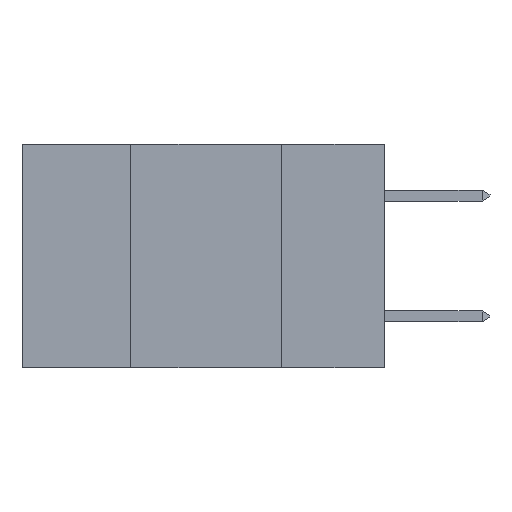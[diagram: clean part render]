
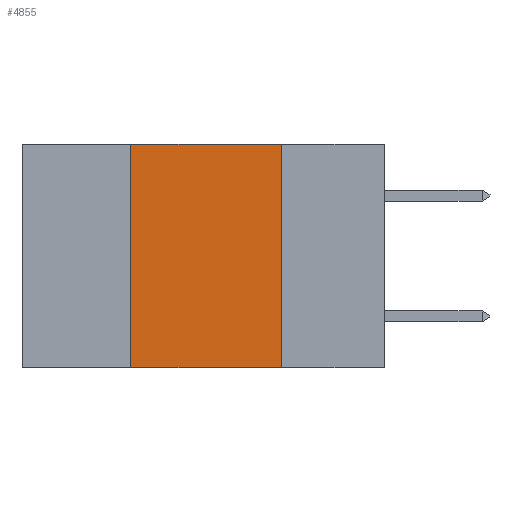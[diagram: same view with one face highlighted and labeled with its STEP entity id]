
A CAD part, left-side view. The second image highlights one B-rep face of the part: STEP entity #4855.
In plain terms, the highlighted planar face has unit normal (-1, 0, 0).
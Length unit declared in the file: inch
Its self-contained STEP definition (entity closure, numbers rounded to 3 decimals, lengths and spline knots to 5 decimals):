
#382 = CARTESIAN_POINT ( 'NONE',  ( 0., 0.42, -0.37 ) ) ;
#876 = VECTOR ( 'NONE', #8269, 39.37008 ) ;
#1705 = AXIS2_PLACEMENT_3D ( 'NONE', #3539, #5589, #12996 ) ;
#2665 = EDGE_CURVE ( 'NONE', #5939, #7210, #4431, .T. ) ;
#2969 = ORIENTED_EDGE ( 'NONE', *, *, #2665, .F. ) ;
#3015 = ORIENTED_EDGE ( 'NONE', *, *, #3837, .F. ) ;
#3060 = ORIENTED_EDGE ( 'NONE', *, *, #10704, .F. ) ;
#3158 = ORIENTED_EDGE ( 'NONE', *, *, #7846, .T. ) ;
#3539 = CARTESIAN_POINT ( 'NONE',  ( 0., 0.6, 0. ) ) ;
#3681 = LINE ( 'NONE', #5113, #876 ) ;
#3837 = EDGE_CURVE ( 'NONE', #6225, #5939, #9857, .T. ) ;
#4431 = LINE ( 'NONE', #7300, #12510 ) ;
#4486 = CARTESIAN_POINT ( 'NONE',  ( 0., 0.42, 0. ) ) ;
#4662 = EDGE_LOOP ( 'NONE', ( #2969, #3015, #3060, #3158 ) ) ;
#4855 = ADVANCED_FACE ( 'NONE', ( #6745 ), #8763, .F. ) ;
#4867 = VERTEX_POINT ( 'NONE', #382 ) ;
#4898 = CARTESIAN_POINT ( 'NONE',  ( 0., 0.6, -0.37 ) ) ;
#5001 = CARTESIAN_POINT ( 'NONE',  ( 0., 0.6, 0. ) ) ;
#5077 = CARTESIAN_POINT ( 'NONE',  ( 0., 0.17, 0. ) ) ;
#5113 = CARTESIAN_POINT ( 'NONE',  ( 0., 0.42, 0. ) ) ;
#5589 = DIRECTION ( 'NONE',  ( 1., 0., 0. ) ) ;
#5805 = LINE ( 'NONE', #4898, #13520 ) ;
#5939 = VERTEX_POINT ( 'NONE', #5077 ) ;
#6225 = VERTEX_POINT ( 'NONE', #4486 ) ;
#6745 = FACE_OUTER_BOUND ( 'NONE', #4662, .T. ) ;
#7009 = DIRECTION ( 'NONE',  ( 0., -1., 0. ) ) ;
#7025 = VECTOR ( 'NONE', #7124, 39.37008 ) ;
#7124 = DIRECTION ( 'NONE',  ( 0., -1., 0. ) ) ;
#7210 = VERTEX_POINT ( 'NONE', #8091 ) ;
#7300 = CARTESIAN_POINT ( 'NONE',  ( 0., 0.17, 0. ) ) ;
#7846 = EDGE_CURVE ( 'NONE', #4867, #7210, #5805, .T. ) ;
#8091 = CARTESIAN_POINT ( 'NONE',  ( 0., 0.17, -0.37 ) ) ;
#8269 = DIRECTION ( 'NONE',  ( 0., 0., 1. ) ) ;
#8763 = PLANE ( 'NONE',  #1705 ) ;
#9857 = LINE ( 'NONE', #5001, #7025 ) ;
#10704 = EDGE_CURVE ( 'NONE', #4867, #6225, #3681, .T. ) ;
#11554 = DIRECTION ( 'NONE',  ( 0., 0., -1. ) ) ;
#12510 = VECTOR ( 'NONE', #11554, 39.37008 ) ;
#12996 = DIRECTION ( 'NONE',  ( 0., 0., -1. ) ) ;
#13520 = VECTOR ( 'NONE', #7009, 39.37008 ) ;
